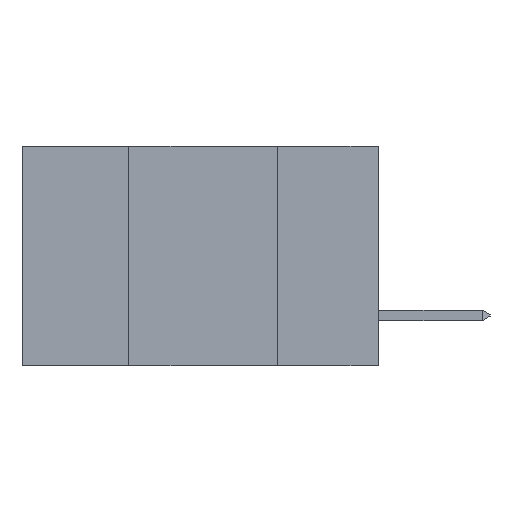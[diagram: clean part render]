
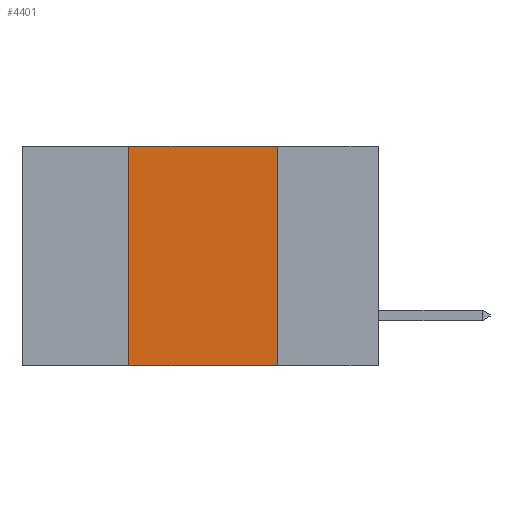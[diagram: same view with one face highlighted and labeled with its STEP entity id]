
A CAD part, left-side view. The second image highlights one B-rep face of the part: STEP entity #4401.
In plain terms, the highlighted planar face has unit normal (-1, 0, 0).
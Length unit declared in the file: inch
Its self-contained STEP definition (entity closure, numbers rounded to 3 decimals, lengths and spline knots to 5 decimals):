
#385 = EDGE_CURVE ( 'NONE', #10129, #770, #13990, .T. ) ;
#770 = VERTEX_POINT ( 'NONE', #8532 ) ;
#1085 = CARTESIAN_POINT ( 'NONE',  ( 0., 0.17, -0.37 ) ) ;
#2117 = VECTOR ( 'NONE', #14741, 39.37008 ) ;
#3095 = VERTEX_POINT ( 'NONE', #1085 ) ;
#3302 = DIRECTION ( 'NONE',  ( 0., -1., 0. ) ) ;
#3989 = VECTOR ( 'NONE', #3302, 39.37008 ) ;
#4056 = CARTESIAN_POINT ( 'NONE',  ( 0., 0.6, 0. ) ) ;
#4084 = EDGE_CURVE ( 'NONE', #770, #7188, #9856, .T. ) ;
#4401 = ADVANCED_FACE ( 'NONE', ( #15424 ), #12156, .F. ) ;
#4407 = LINE ( 'NONE', #7431, #3989 ) ;
#5014 = EDGE_CURVE ( 'NONE', #7188, #3095, #12946, .T. ) ;
#5341 = CARTESIAN_POINT ( 'NONE',  ( 0., 0.17, -0.37 ) ) ;
#5440 = DIRECTION ( 'NONE',  ( 1., 0., 0. ) ) ;
#5797 = DIRECTION ( 'NONE',  ( 0., 0., 1. ) ) ;
#7188 = VERTEX_POINT ( 'NONE', #9980 ) ;
#7431 = CARTESIAN_POINT ( 'NONE',  ( 0., 0.6, -0.37 ) ) ;
#7469 = CARTESIAN_POINT ( 'NONE',  ( 0., 0.42, -0.37 ) ) ;
#8532 = CARTESIAN_POINT ( 'NONE',  ( 0., 0.42, 0. ) ) ;
#9856 = LINE ( 'NONE', #14144, #12984 ) ;
#9912 = EDGE_LOOP ( 'NONE', ( #11909, #13649, #10723, #12819 ) ) ;
#9980 = CARTESIAN_POINT ( 'NONE',  ( 0., 0.17, 0. ) ) ;
#10129 = VERTEX_POINT ( 'NONE', #13052 ) ;
#10723 = ORIENTED_EDGE ( 'NONE', *, *, #385, .F. ) ;
#11909 = ORIENTED_EDGE ( 'NONE', *, *, #5014, .F. ) ;
#12156 = PLANE ( 'NONE',  #12357 ) ;
#12357 = AXIS2_PLACEMENT_3D ( 'NONE', #4056, #5440, #14833 ) ;
#12819 = ORIENTED_EDGE ( 'NONE', *, *, #16998, .T. ) ;
#12946 = LINE ( 'NONE', #5341, #2117 ) ;
#12984 = VECTOR ( 'NONE', #15512, 39.37008 ) ;
#13052 = CARTESIAN_POINT ( 'NONE',  ( 0., 0.42, -0.37 ) ) ;
#13649 = ORIENTED_EDGE ( 'NONE', *, *, #4084, .F. ) ;
#13990 = LINE ( 'NONE', #7469, #14823 ) ;
#14144 = CARTESIAN_POINT ( 'NONE',  ( 0., 0.6, 0. ) ) ;
#14741 = DIRECTION ( 'NONE',  ( 0., 0., -1. ) ) ;
#14823 = VECTOR ( 'NONE', #5797, 39.37008 ) ;
#14833 = DIRECTION ( 'NONE',  ( 0., 0., -1. ) ) ;
#15424 = FACE_OUTER_BOUND ( 'NONE', #9912, .T. ) ;
#15512 = DIRECTION ( 'NONE',  ( 0., -1., 0. ) ) ;
#16998 = EDGE_CURVE ( 'NONE', #10129, #3095, #4407, .T. ) ;
